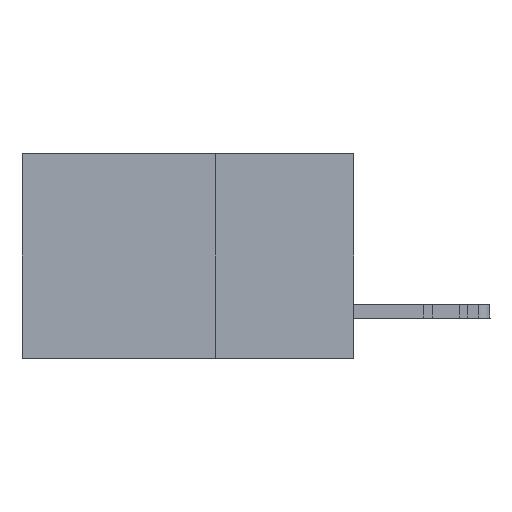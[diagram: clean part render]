
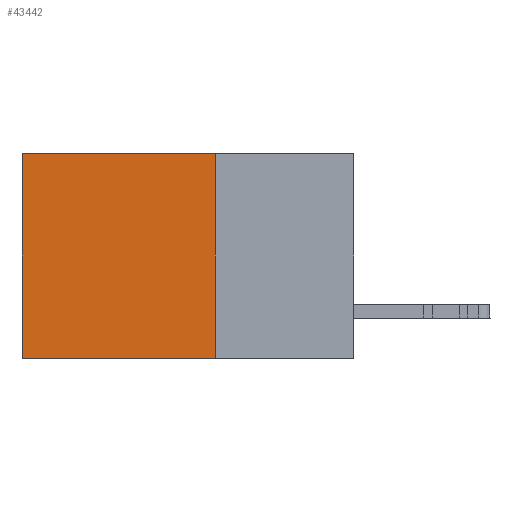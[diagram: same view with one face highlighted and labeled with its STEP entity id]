
A CAD part, left-side view. The second image highlights one B-rep face of the part: STEP entity #43442.
In plain terms, the highlighted planar face has unit normal (-1, 0, 0).
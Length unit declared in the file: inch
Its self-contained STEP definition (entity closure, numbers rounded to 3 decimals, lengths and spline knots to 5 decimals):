
#2837 = EDGE_CURVE ( 'NONE', #8550, #11796, #12122, .T. ) ;
#3712 = VECTOR ( 'NONE', #25543, 39.37008 ) ;
#5409 = AXIS2_PLACEMENT_3D ( 'NONE', #20381, #26877, #13420 ) ;
#6335 = ORIENTED_EDGE ( 'NONE', *, *, #2837, .F. ) ;
#8550 = VERTEX_POINT ( 'NONE', #38108 ) ;
#9463 = CARTESIAN_POINT ( 'NONE',  ( 0.2875, 0.25, 0. ) ) ;
#9487 = LINE ( 'NONE', #41059, #21117 ) ;
#10478 = VERTEX_POINT ( 'NONE', #27854 ) ;
#11796 = VERTEX_POINT ( 'NONE', #19366 ) ;
#12122 = LINE ( 'NONE', #16694, #32062 ) ;
#13420 = DIRECTION ( 'NONE',  ( 0., 0., -1. ) ) ;
#14726 = CARTESIAN_POINT ( 'NONE',  ( 0.2875, 0.25, 0. ) ) ;
#15090 = VECTOR ( 'NONE', #24458, 39.37008 ) ;
#16694 = CARTESIAN_POINT ( 'NONE',  ( 0.2875, 0.25, -0.37 ) ) ;
#17274 = CARTESIAN_POINT ( 'NONE',  ( 0.2875, 0.6, 0. ) ) ;
#18356 = ORIENTED_EDGE ( 'NONE', *, *, #27112, .T. ) ;
#19363 = FACE_OUTER_BOUND ( 'NONE', #21148, .T. ) ;
#19366 = CARTESIAN_POINT ( 'NONE',  ( 0.2875, 0.6, -0.37 ) ) ;
#20381 = CARTESIAN_POINT ( 'NONE',  ( 0.2875, 0.25, 0. ) ) ;
#21117 = VECTOR ( 'NONE', #40905, 39.37008 ) ;
#21148 = EDGE_LOOP ( 'NONE', ( #18356, #6335, #31262, #29883 ) ) ;
#22339 = EDGE_CURVE ( 'NONE', #10478, #8550, #39999, .T. ) ;
#23631 = PLANE ( 'NONE',  #5409 ) ;
#23914 = EDGE_CURVE ( 'NONE', #10478, #24225, #42845, .T. ) ;
#24225 = VERTEX_POINT ( 'NONE', #17274 ) ;
#24458 = DIRECTION ( 'NONE',  ( 0., 0., -1. ) ) ;
#25543 = DIRECTION ( 'NONE',  ( 0., 1., 0. ) ) ;
#26877 = DIRECTION ( 'NONE',  ( 1., 0., 0. ) ) ;
#27112 = EDGE_CURVE ( 'NONE', #24225, #11796, #9487, .T. ) ;
#27854 = CARTESIAN_POINT ( 'NONE',  ( 0.2875, 0.25, 0. ) ) ;
#29883 = ORIENTED_EDGE ( 'NONE', *, *, #23914, .T. ) ;
#31262 = ORIENTED_EDGE ( 'NONE', *, *, #22339, .F. ) ;
#32062 = VECTOR ( 'NONE', #41364, 39.37008 ) ;
#38108 = CARTESIAN_POINT ( 'NONE',  ( 0.2875, 0.25, -0.37 ) ) ;
#39999 = LINE ( 'NONE', #9463, #15090 ) ;
#40905 = DIRECTION ( 'NONE',  ( 0., 0., -1. ) ) ;
#41059 = CARTESIAN_POINT ( 'NONE',  ( 0.2875, 0.6, 0. ) ) ;
#41364 = DIRECTION ( 'NONE',  ( 0., 1., 0. ) ) ;
#42845 = LINE ( 'NONE', #14726, #3712 ) ;
#43442 = ADVANCED_FACE ( 'NONE', ( #19363 ), #23631, .F. ) ;
